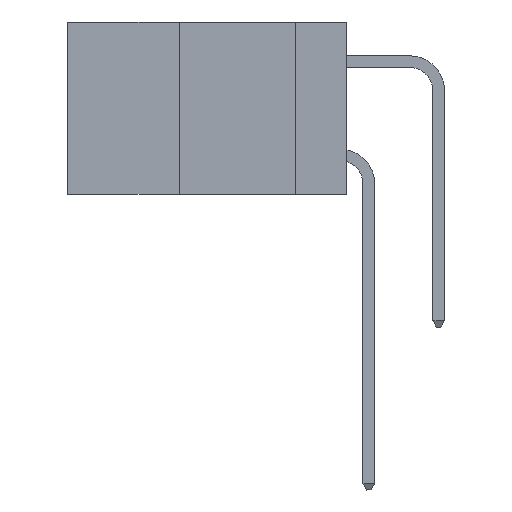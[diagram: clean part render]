
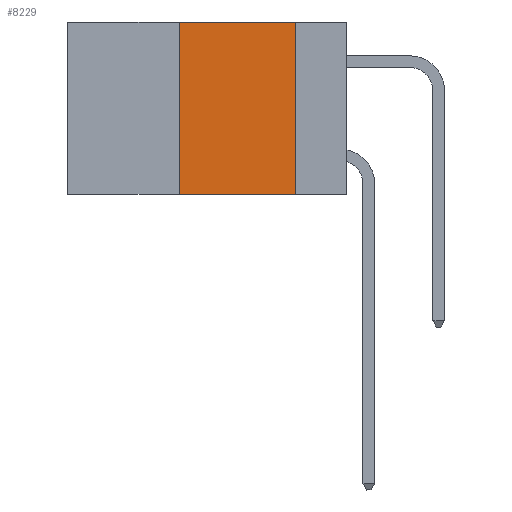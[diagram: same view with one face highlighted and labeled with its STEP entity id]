
A CAD part, left-side view. The second image highlights one B-rep face of the part: STEP entity #8229.
In plain terms, the highlighted planar face has unit normal (-1, 0, 0).
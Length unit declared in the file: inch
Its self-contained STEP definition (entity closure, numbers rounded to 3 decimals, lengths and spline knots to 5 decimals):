
#117 = ORIENTED_EDGE ( 'NONE', *, *, #3243, .F. ) ;
#166 = FACE_OUTER_BOUND ( 'NONE', #19888, .T. ) ;
#470 = LINE ( 'NONE', #2599, #4203 ) ;
#496 = AXIS2_PLACEMENT_3D ( 'NONE', #12516, #2741, #4871 ) ;
#1126 = VERTEX_POINT ( 'NONE', #15851 ) ;
#1794 = ORIENTED_EDGE ( 'NONE', *, *, #3760, .T. ) ;
#2042 = ORIENTED_EDGE ( 'NONE', *, *, #23422, .F. ) ;
#2599 = CARTESIAN_POINT ( 'NONE',  ( 0., 0.36, 0. ) ) ;
#2741 = DIRECTION ( 'NONE',  ( 1., 0., 0. ) ) ;
#3021 = CARTESIAN_POINT ( 'NONE',  ( 0., 0.11, 0. ) ) ;
#3243 = EDGE_CURVE ( 'NONE', #18999, #1126, #18993, .T. ) ;
#3760 = EDGE_CURVE ( 'NONE', #16678, #1126, #20329, .T. ) ;
#4203 = VECTOR ( 'NONE', #18126, 39.37008 ) ;
#4871 = DIRECTION ( 'NONE',  ( 0., 0., -1. ) ) ;
#6484 = DIRECTION ( 'NONE',  ( 0., -1., 0. ) ) ;
#8229 = ADVANCED_FACE ( 'NONE', ( #166 ), #10602, .F. ) ;
#9590 = ORIENTED_EDGE ( 'NONE', *, *, #24903, .F. ) ;
#9663 = DIRECTION ( 'NONE',  ( 0., 0., -1. ) ) ;
#10602 = PLANE ( 'NONE',  #496 ) ;
#10732 = CARTESIAN_POINT ( 'NONE',  ( 0., 0.6, 0. ) ) ;
#12222 = VECTOR ( 'NONE', #9663, 39.37008 ) ;
#12516 = CARTESIAN_POINT ( 'NONE',  ( 0., 0.6, 0. ) ) ;
#12817 = VECTOR ( 'NONE', #6484, 39.37008 ) ;
#15047 = CARTESIAN_POINT ( 'NONE',  ( 0., 0.36, 0. ) ) ;
#15406 = VECTOR ( 'NONE', #16505, 39.37008 ) ;
#15851 = CARTESIAN_POINT ( 'NONE',  ( 0., 0.11, -0.37 ) ) ;
#16466 = LINE ( 'NONE', #10732, #12817 ) ;
#16505 = DIRECTION ( 'NONE',  ( 0., -1., 0. ) ) ;
#16678 = VERTEX_POINT ( 'NONE', #18986 ) ;
#18126 = DIRECTION ( 'NONE',  ( 0., 0., 1. ) ) ;
#18384 = VERTEX_POINT ( 'NONE', #15047 ) ;
#18986 = CARTESIAN_POINT ( 'NONE',  ( 0., 0.36, -0.37 ) ) ;
#18993 = LINE ( 'NONE', #23382, #12222 ) ;
#18999 = VERTEX_POINT ( 'NONE', #3021 ) ;
#19888 = EDGE_LOOP ( 'NONE', ( #117, #9590, #2042, #1794 ) ) ;
#20329 = LINE ( 'NONE', #24555, #15406 ) ;
#23382 = CARTESIAN_POINT ( 'NONE',  ( 0., 0.11, 0. ) ) ;
#23422 = EDGE_CURVE ( 'NONE', #16678, #18384, #470, .T. ) ;
#24555 = CARTESIAN_POINT ( 'NONE',  ( 0., 0.6, -0.37 ) ) ;
#24903 = EDGE_CURVE ( 'NONE', #18384, #18999, #16466, .T. ) ;
